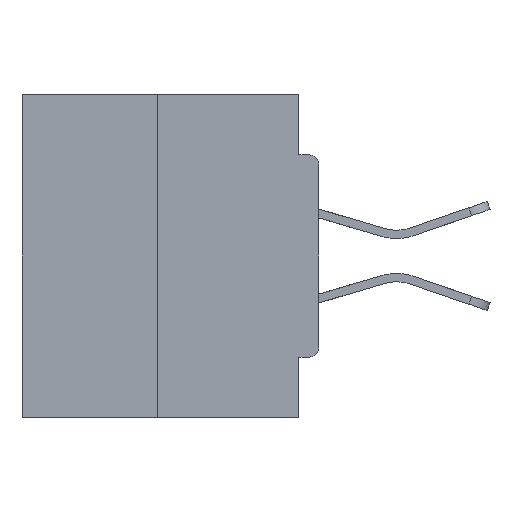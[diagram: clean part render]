
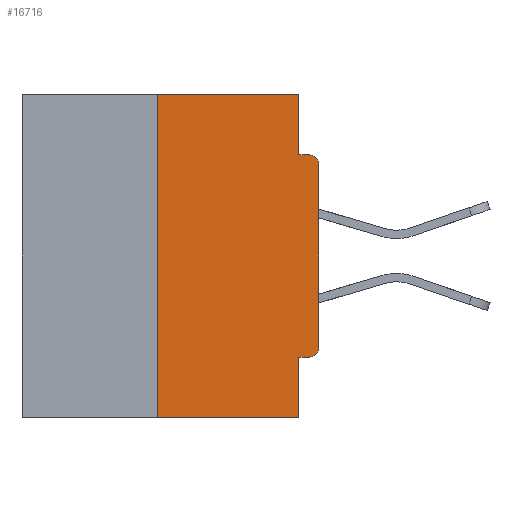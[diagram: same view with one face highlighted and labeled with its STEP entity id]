
A CAD part, left-side view. The second image highlights one B-rep face of the part: STEP entity #16716.
In plain terms, the highlighted planar face has unit normal (-1, 0, 0).
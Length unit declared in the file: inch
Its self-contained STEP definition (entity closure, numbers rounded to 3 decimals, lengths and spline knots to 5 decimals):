
#721 = ORIENTED_EDGE ( 'NONE', *, *, #16594, .F. ) ;
#1630 = EDGE_CURVE ( 'NONE', #9621, #16067, #8771, .T. ) ;
#1957 = LINE ( 'NONE', #12619, #9693 ) ;
#1979 = VERTEX_POINT ( 'NONE', #11464 ) ;
#2001 = CARTESIAN_POINT ( 'NONE',  ( 0., 0., -0.0935 ) ) ;
#2033 = DIRECTION ( 'NONE',  ( 0., 1., 0. ) ) ;
#2465 = DIRECTION ( 'NONE',  ( 0., 0., 1. ) ) ;
#3807 = EDGE_CURVE ( 'NONE', #26516, #29413, #25330, .T. ) ;
#4513 = DIRECTION ( 'NONE',  ( 0., -1., 0. ) ) ;
#5213 = LINE ( 'NONE', #20440, #10479 ) ;
#5356 = DIRECTION ( 'NONE',  ( 1., 0., 0. ) ) ;
#5539 = CARTESIAN_POINT ( 'NONE',  ( 0., 0.25, 0. ) ) ;
#6071 = VECTOR ( 'NONE', #2033, 39.37008 ) ;
#6488 = ORIENTED_EDGE ( 'NONE', *, *, #3807, .F. ) ;
#6645 = CIRCLE ( 'NONE', #24394, 0.015 ) ;
#7616 = VERTEX_POINT ( 'NONE', #17906 ) ;
#8131 = AXIS2_PLACEMENT_3D ( 'NONE', #30463, #14667, #33093 ) ;
#8385 = EDGE_CURVE ( 'NONE', #26516, #16067, #25472, .T. ) ;
#8427 = FACE_OUTER_BOUND ( 'NONE', #21003, .T. ) ;
#8771 = LINE ( 'NONE', #24975, #16879 ) ;
#9621 = VERTEX_POINT ( 'NONE', #21080 ) ;
#9693 = VECTOR ( 'NONE', #33756, 39.37008 ) ;
#10479 = VECTOR ( 'NONE', #2465, 39.37008 ) ;
#11464 = CARTESIAN_POINT ( 'NONE',  ( 0., 0., -0.1085 ) ) ;
#11715 = DIRECTION ( 'NONE',  ( 0., 0., -1. ) ) ;
#12619 = CARTESIAN_POINT ( 'NONE',  ( 0., 0.46, 0. ) ) ;
#13147 = CARTESIAN_POINT ( 'NONE',  ( 0., 0.46, 0. ) ) ;
#14171 = CARTESIAN_POINT ( 'NONE',  ( 0., 0.25, 0. ) ) ;
#14659 = EDGE_CURVE ( 'NONE', #7616, #18821, #14694, .T. ) ;
#14667 = DIRECTION ( 'NONE',  ( -1., 0., 0. ) ) ;
#14694 = CIRCLE ( 'NONE', #8131, 0.015 ) ;
#15070 = CARTESIAN_POINT ( 'NONE',  ( 0., 0., -0.4065 ) ) ;
#16067 = VERTEX_POINT ( 'NONE', #21916 ) ;
#16267 = DIRECTION ( 'NONE',  ( 0., 0., -1. ) ) ;
#16594 = EDGE_CURVE ( 'NONE', #29413, #32384, #1957, .T. ) ;
#16620 = CARTESIAN_POINT ( 'NONE',  ( 0., 0.031, -0.0935 ) ) ;
#16641 = CARTESIAN_POINT ( 'NONE',  ( 0., 0.031, 0. ) ) ;
#16650 = VERTEX_POINT ( 'NONE', #28471 ) ;
#16716 = ADVANCED_FACE ( 'NONE', ( #8427 ), #20802, .F. ) ;
#16838 = ORIENTED_EDGE ( 'NONE', *, *, #1630, .F. ) ;
#16879 = VECTOR ( 'NONE', #25430, 39.37008 ) ;
#17283 = ORIENTED_EDGE ( 'NONE', *, *, #26590, .F. ) ;
#17402 = VERTEX_POINT ( 'NONE', #16620 ) ;
#17789 = ORIENTED_EDGE ( 'NONE', *, *, #28659, .F. ) ;
#17906 = CARTESIAN_POINT ( 'NONE',  ( 0., 0.015, -0.4065 ) ) ;
#17973 = VECTOR ( 'NONE', #11715, 39.37008 ) ;
#18164 = DIRECTION ( 'NONE',  ( 0., 0., -1. ) ) ;
#18821 = VERTEX_POINT ( 'NONE', #30728 ) ;
#19550 = CARTESIAN_POINT ( 'NONE',  ( 0., 0.031, 0. ) ) ;
#19869 = LINE ( 'NONE', #15070, #6071 ) ;
#20440 = CARTESIAN_POINT ( 'NONE',  ( 0., 0., 0. ) ) ;
#20802 = PLANE ( 'NONE',  #22359 ) ;
#21003 = EDGE_LOOP ( 'NONE', ( #721, #6488, #30653, #16838, #17789, #28004, #32146, #21249, #24594, #17283 ) ) ;
#21046 = LINE ( 'NONE', #2001, #30512 ) ;
#21080 = CARTESIAN_POINT ( 'NONE',  ( 0., 0.031, -0.4065 ) ) ;
#21102 = DIRECTION ( 'NONE',  ( 0., 0., 1. ) ) ;
#21249 = ORIENTED_EDGE ( 'NONE', *, *, #25987, .T. ) ;
#21391 = VECTOR ( 'NONE', #4513, 39.37008 ) ;
#21658 = DIRECTION ( 'NONE',  ( -1., 0., 0. ) ) ;
#21916 = CARTESIAN_POINT ( 'NONE',  ( 0., 0.031, -0.5 ) ) ;
#22083 = LINE ( 'NONE', #19550, #17973 ) ;
#22359 = AXIS2_PLACEMENT_3D ( 'NONE', #13147, #5356, #18164 ) ;
#23163 = CARTESIAN_POINT ( 'NONE',  ( 0., 0.46, -0.5 ) ) ;
#24141 = CARTESIAN_POINT ( 'NONE',  ( 0., 0.25, -0.5 ) ) ;
#24394 = AXIS2_PLACEMENT_3D ( 'NONE', #26958, #21658, #16267 ) ;
#24507 = VECTOR ( 'NONE', #21102, 39.37008 ) ;
#24594 = ORIENTED_EDGE ( 'NONE', *, *, #28880, .F. ) ;
#24975 = CARTESIAN_POINT ( 'NONE',  ( 0., 0.031, -0.5 ) ) ;
#25330 = LINE ( 'NONE', #5539, #24507 ) ;
#25430 = DIRECTION ( 'NONE',  ( 0., 0., -1. ) ) ;
#25472 = LINE ( 'NONE', #23163, #21391 ) ;
#25987 = EDGE_CURVE ( 'NONE', #1979, #16650, #6645, .T. ) ;
#26516 = VERTEX_POINT ( 'NONE', #24141 ) ;
#26590 = EDGE_CURVE ( 'NONE', #32384, #17402, #22083, .T. ) ;
#26958 = CARTESIAN_POINT ( 'NONE',  ( 0., 0.015, -0.1085 ) ) ;
#28004 = ORIENTED_EDGE ( 'NONE', *, *, #14659, .T. ) ;
#28471 = CARTESIAN_POINT ( 'NONE',  ( 0., 0.015, -0.0935 ) ) ;
#28659 = EDGE_CURVE ( 'NONE', #7616, #9621, #19869, .T. ) ;
#28880 = EDGE_CURVE ( 'NONE', #17402, #16650, #21046, .T. ) ;
#29413 = VERTEX_POINT ( 'NONE', #14171 ) ;
#30463 = CARTESIAN_POINT ( 'NONE',  ( 0., 0.015, -0.3915 ) ) ;
#30512 = VECTOR ( 'NONE', #33592, 39.37008 ) ;
#30653 = ORIENTED_EDGE ( 'NONE', *, *, #8385, .T. ) ;
#30728 = CARTESIAN_POINT ( 'NONE',  ( 0., 0., -0.3915 ) ) ;
#32130 = EDGE_CURVE ( 'NONE', #18821, #1979, #5213, .T. ) ;
#32146 = ORIENTED_EDGE ( 'NONE', *, *, #32130, .T. ) ;
#32384 = VERTEX_POINT ( 'NONE', #16641 ) ;
#33093 = DIRECTION ( 'NONE',  ( 0., 0., -1. ) ) ;
#33592 = DIRECTION ( 'NONE',  ( 0., -1., 0. ) ) ;
#33756 = DIRECTION ( 'NONE',  ( 0., -1., 0. ) ) ;
